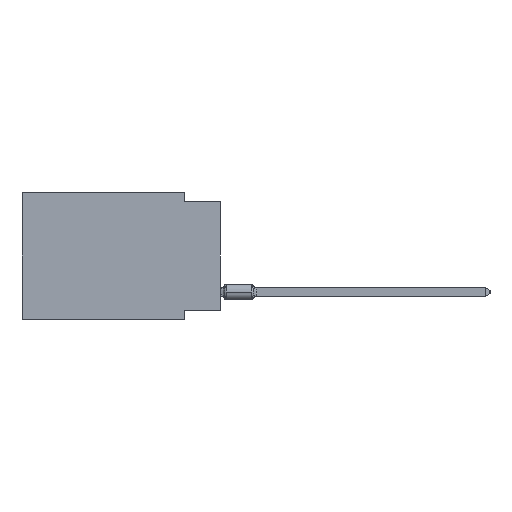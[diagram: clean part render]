
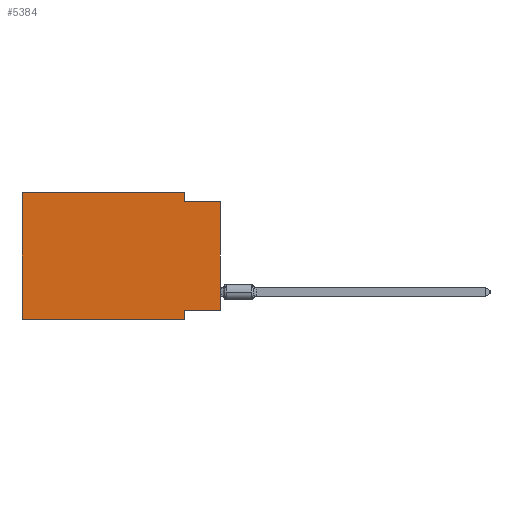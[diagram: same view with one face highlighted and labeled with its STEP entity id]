
A CAD part, left-side view. The second image highlights one B-rep face of the part: STEP entity #5384.
In plain terms, the highlighted planar face has unit normal (-1, 0, 0).
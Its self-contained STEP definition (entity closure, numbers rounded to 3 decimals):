
#165 = DIRECTION ( 'NONE',  ( 0., 0., -1. ) ) ;
#1980 = VERTEX_POINT ( 'NONE', #31684 ) ;
#2253 = DIRECTION ( 'NONE',  ( 0., 0., -1. ) ) ;
#2663 = CARTESIAN_POINT ( 'NONE',  ( 0., 2.54, -8.89 ) ) ;
#2849 = CARTESIAN_POINT ( 'NONE',  ( 0., 2.54, 0. ) ) ;
#5384 = ADVANCED_FACE ( 'NONE', ( #16079 ), #7294, .F. ) ;
#6209 = ORIENTED_EDGE ( 'NONE', *, *, #15684, .T. ) ;
#6619 = DIRECTION ( 'NONE',  ( 0., 1., 0. ) ) ;
#7294 = PLANE ( 'NONE',  #34545 ) ;
#7482 = EDGE_CURVE ( 'NONE', #31132, #13104, #10326, .T. ) ;
#7761 = DIRECTION ( 'NONE',  ( 0., -1., 0. ) ) ;
#7939 = VECTOR ( 'NONE', #9587, 1000. ) ;
#8758 = CARTESIAN_POINT ( 'NONE',  ( 0., 13.97, 0. ) ) ;
#9130 = VERTEX_POINT ( 'NONE', #38471 ) ;
#9520 = DIRECTION ( 'NONE',  ( 0., 0., 1. ) ) ;
#9587 = DIRECTION ( 'NONE',  ( 0., -1., 0. ) ) ;
#10326 = LINE ( 'NONE', #29728, #21336 ) ;
#12202 = ORIENTED_EDGE ( 'NONE', *, *, #34301, .F. ) ;
#12306 = LINE ( 'NONE', #21898, #7939 ) ;
#12727 = CARTESIAN_POINT ( 'NONE',  ( 0., 13.97, 0. ) ) ;
#13104 = VERTEX_POINT ( 'NONE', #21187 ) ;
#13260 = LINE ( 'NONE', #25382, #35353 ) ;
#14824 = VECTOR ( 'NONE', #165, 1000. ) ;
#15680 = VERTEX_POINT ( 'NONE', #41254 ) ;
#15684 = EDGE_CURVE ( 'NONE', #33029, #1980, #13260, .T. ) ;
#16079 = FACE_OUTER_BOUND ( 'NONE', #35925, .T. ) ;
#17799 = CARTESIAN_POINT ( 'NONE',  ( 0., 0., -0.635 ) ) ;
#17999 = VERTEX_POINT ( 'NONE', #37427 ) ;
#18126 = LINE ( 'NONE', #2849, #38895 ) ;
#19718 = DIRECTION ( 'NONE',  ( 0., -1., 0. ) ) ;
#20032 = CARTESIAN_POINT ( 'NONE',  ( 0., 13.97, 0. ) ) ;
#20540 = ORIENTED_EDGE ( 'NONE', *, *, #28683, .F. ) ;
#20676 = EDGE_CURVE ( 'NONE', #31132, #25403, #31121, .T. ) ;
#21187 = CARTESIAN_POINT ( 'NONE',  ( 0., 2.54, -8.89 ) ) ;
#21336 = VECTOR ( 'NONE', #19718, 1000. ) ;
#21898 = CARTESIAN_POINT ( 'NONE',  ( 0., 13.97, 0. ) ) ;
#23660 = VECTOR ( 'NONE', #6619, 1000. ) ;
#25382 = CARTESIAN_POINT ( 'NONE',  ( 0., 0., 0. ) ) ;
#25403 = VERTEX_POINT ( 'NONE', #8758 ) ;
#25613 = ORIENTED_EDGE ( 'NONE', *, *, #39324, .F. ) ;
#25716 = EDGE_CURVE ( 'NONE', #9130, #17999, #18126, .T. ) ;
#25995 = ORIENTED_EDGE ( 'NONE', *, *, #20676, .F. ) ;
#26909 = CARTESIAN_POINT ( 'NONE',  ( 0., 0., -8.255 ) ) ;
#28197 = VECTOR ( 'NONE', #34459, 1000. ) ;
#28683 = EDGE_CURVE ( 'NONE', #33029, #15680, #31875, .T. ) ;
#28748 = CARTESIAN_POINT ( 'NONE',  ( 0., 0., -8.255 ) ) ;
#28756 = LINE ( 'NONE', #2663, #14824 ) ;
#29728 = CARTESIAN_POINT ( 'NONE',  ( 0., 13.97, -8.89 ) ) ;
#31121 = LINE ( 'NONE', #12727, #28197 ) ;
#31132 = VERTEX_POINT ( 'NONE', #32809 ) ;
#31684 = CARTESIAN_POINT ( 'NONE',  ( 0., 0., -0.635 ) ) ;
#31775 = EDGE_CURVE ( 'NONE', #15680, #13104, #28756, .T. ) ;
#31875 = LINE ( 'NONE', #28748, #23660 ) ;
#31934 = DIRECTION ( 'NONE',  ( 0., 0., -1. ) ) ;
#32809 = CARTESIAN_POINT ( 'NONE',  ( 0., 13.97, -8.89 ) ) ;
#33029 = VERTEX_POINT ( 'NONE', #26909 ) ;
#34301 = EDGE_CURVE ( 'NONE', #17999, #1980, #36572, .T. ) ;
#34459 = DIRECTION ( 'NONE',  ( 0., 0., 1. ) ) ;
#34545 = AXIS2_PLACEMENT_3D ( 'NONE', #20032, #38831, #31934 ) ;
#35353 = VECTOR ( 'NONE', #9520, 1000. ) ;
#35925 = EDGE_LOOP ( 'NONE', ( #6209, #12202, #36100, #25613, #25995, #41183, #38245, #20540 ) ) ;
#36100 = ORIENTED_EDGE ( 'NONE', *, *, #25716, .F. ) ;
#36572 = LINE ( 'NONE', #17799, #40031 ) ;
#37427 = CARTESIAN_POINT ( 'NONE',  ( 0., 2.54, -0.635 ) ) ;
#38245 = ORIENTED_EDGE ( 'NONE', *, *, #31775, .F. ) ;
#38471 = CARTESIAN_POINT ( 'NONE',  ( 0., 2.54, 0. ) ) ;
#38831 = DIRECTION ( 'NONE',  ( 1., 0., 0. ) ) ;
#38895 = VECTOR ( 'NONE', #2253, 1000. ) ;
#39324 = EDGE_CURVE ( 'NONE', #25403, #9130, #12306, .T. ) ;
#40031 = VECTOR ( 'NONE', #7761, 1000. ) ;
#41183 = ORIENTED_EDGE ( 'NONE', *, *, #7482, .T. ) ;
#41254 = CARTESIAN_POINT ( 'NONE',  ( 0., 2.54, -8.255 ) ) ;
